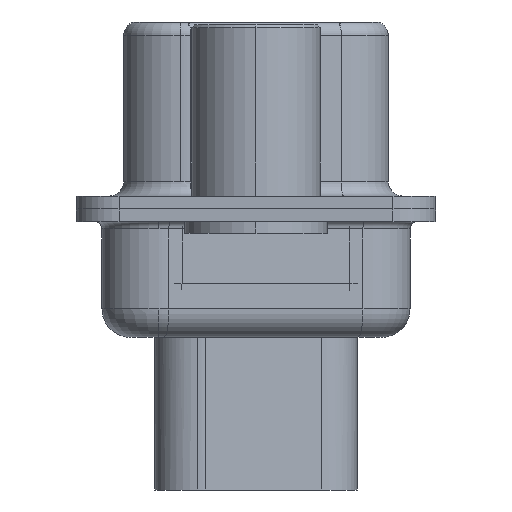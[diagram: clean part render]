
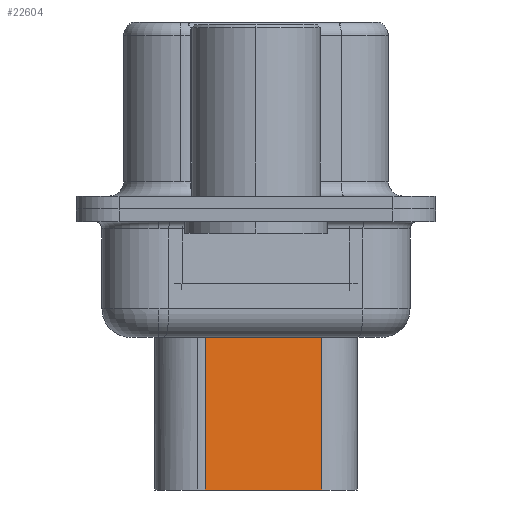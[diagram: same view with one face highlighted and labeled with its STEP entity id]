
A CAD part, left-side view. The second image highlights one B-rep face of the part: STEP entity #22604.
In plain terms, the highlighted planar face has unit normal (-0.985, -0.174, 0).
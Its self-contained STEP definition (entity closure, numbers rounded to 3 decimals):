
#541 = CARTESIAN_POINT ( 'NONE',  ( 4.524, 1.78, -9.85 ) ) ;
#1273 = VECTOR ( 'NONE', #11744, 1000. ) ;
#1436 = VECTOR ( 'NONE', #22159, 1000. ) ;
#2230 = LINE ( 'NONE', #4559, #1436 ) ;
#2404 = ORIENTED_EDGE ( 'NONE', *, *, #13283, .F. ) ;
#3612 = CARTESIAN_POINT ( 'NONE',  ( 4.524, 1.78, -3.1 ) ) ;
#4559 = CARTESIAN_POINT ( 'NONE',  ( 4.353, 2.749, -3.975 ) ) ;
#6098 = CARTESIAN_POINT ( 'NONE',  ( 5.243, -2.3, -3.1 ) ) ;
#8518 = FACE_OUTER_BOUND ( 'NONE', #24013, .T. ) ;
#9607 = ORIENTED_EDGE ( 'NONE', *, *, #18032, .T. ) ;
#11744 = DIRECTION ( 'NONE',  ( -0.174, 0.985, 0. ) ) ;
#12753 = PLANE ( 'NONE',  #18238 ) ;
#13155 = ORIENTED_EDGE ( 'NONE', *, *, #27916, .F. ) ;
#13163 = CARTESIAN_POINT ( 'NONE',  ( 5.243, -2.3, -9.85 ) ) ;
#13283 = EDGE_CURVE ( 'NONE', #20298, #17947, #28085, .T. ) ;
#13303 = VERTEX_POINT ( 'NONE', #28225 ) ;
#13315 = LINE ( 'NONE', #28435, #28397 ) ;
#14920 = DIRECTION ( 'NONE',  ( -0.985, -0.174, 0. ) ) ;
#14921 = CARTESIAN_POINT ( 'NONE',  ( 4.524, 1.78, -3.975 ) ) ;
#15926 = VECTOR ( 'NONE', #25765, 1000. ) ;
#16610 = ORIENTED_EDGE ( 'NONE', *, *, #17531, .T. ) ;
#17256 = DIRECTION ( 'NONE',  ( 0.174, -0.985, 0. ) ) ;
#17531 = EDGE_CURVE ( 'NONE', #20298, #25260, #2230, .T. ) ;
#17947 = VERTEX_POINT ( 'NONE', #13163 ) ;
#18032 = EDGE_CURVE ( 'NONE', #25260, #13303, #13315, .T. ) ;
#18238 = AXIS2_PLACEMENT_3D ( 'NONE', #3612, #14920, #17256 ) ;
#18438 = LINE ( 'NONE', #541, #1273 ) ;
#18457 = CARTESIAN_POINT ( 'NONE',  ( 5.243, -2.3, -3.975 ) ) ;
#20298 = VERTEX_POINT ( 'NONE', #18457 ) ;
#22159 = DIRECTION ( 'NONE',  ( -0.174, 0.985, 0. ) ) ;
#22604 = ADVANCED_FACE ( 'NONE', ( #8518 ), #12753, .T. ) ;
#24013 = EDGE_LOOP ( 'NONE', ( #2404, #16610, #9607, #13155 ) ) ;
#25260 = VERTEX_POINT ( 'NONE', #14921 ) ;
#25765 = DIRECTION ( 'NONE',  ( 0., 0., -1. ) ) ;
#26563 = DIRECTION ( 'NONE',  ( 0., 0., -1. ) ) ;
#27916 = EDGE_CURVE ( 'NONE', #17947, #13303, #18438, .T. ) ;
#28085 = LINE ( 'NONE', #6098, #15926 ) ;
#28225 = CARTESIAN_POINT ( 'NONE',  ( 4.524, 1.78, -9.85 ) ) ;
#28397 = VECTOR ( 'NONE', #26563, 1000. ) ;
#28435 = CARTESIAN_POINT ( 'NONE',  ( 4.524, 1.78, -3.1 ) ) ;
